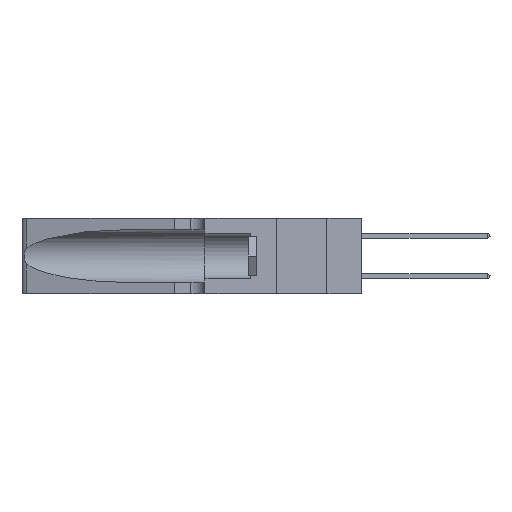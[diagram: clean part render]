
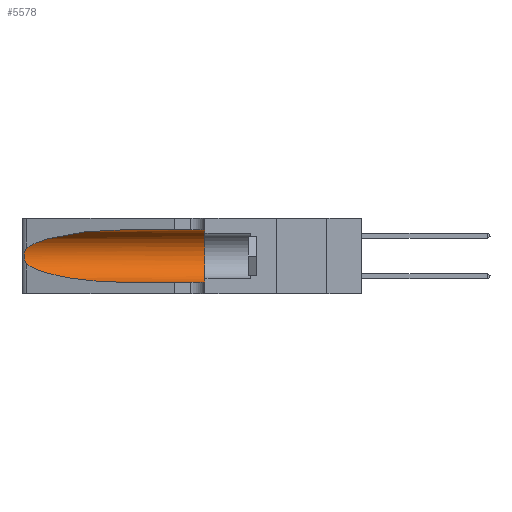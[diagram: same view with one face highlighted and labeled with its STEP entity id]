
A CAD part, left-side view. The second image highlights one B-rep face of the part: STEP entity #5578.
In plain terms, the highlighted cylindrical face has radius 3.308 mm (diameter 6.617 mm), a partial arc.
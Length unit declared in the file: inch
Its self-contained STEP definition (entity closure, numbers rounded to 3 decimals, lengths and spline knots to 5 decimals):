
#259 = CARTESIAN_POINT ( 'NONE',  ( 0.26075, 1.23896, 0.19203 ) ) ;
#334 = VERTEX_POINT ( 'NONE', #24990 ) ;
#492 = CARTESIAN_POINT ( 'NONE',  ( 0.25487, 1.22718, 0.22369 ) ) ;
#1660 = ORIENTED_EDGE ( 'NONE', *, *, #24287, .T. ) ;
#2273 = CARTESIAN_POINT ( 'NONE',  ( 0.25555, 1.22994, 0.2215 ) ) ;
#2366 = CARTESIAN_POINT ( 'NONE',  ( 0.26017, 1.23833, 0.17102 ) ) ;
#2675 = CARTESIAN_POINT ( 'NONE',  ( 0.25487, 1.22718, 0.14631 ) ) ;
#3434 = VERTEX_POINT ( 'NONE', #2675 ) ;
#4401 = CARTESIAN_POINT ( 'NONE',  ( 0.25487, 1.22718, 0.22369 ) ) ;
#4491 = CARTESIAN_POINT ( 'NONE',  ( 0.25789, 1.23486, 0.15765 ) ) ;
#5123 = VECTOR ( 'NONE', #13664, 39.37008 ) ;
#5188 = DIRECTION ( 'NONE',  ( 0., -1., 0. ) ) ;
#5388 = CARTESIAN_POINT ( 'NONE',  ( 0.1305, 0.35, 0.05475 ) ) ;
#5578 = ADVANCED_FACE ( 'NONE', ( #5948 ), #21377, .F. ) ;
#5700 = ORIENTED_EDGE ( 'NONE', *, *, #9911, .T. ) ;
#5877 = VERTEX_POINT ( 'NONE', #492 ) ;
#5948 = FACE_OUTER_BOUND ( 'NONE', #6174, .T. ) ;
#6094 = ORIENTED_EDGE ( 'NONE', *, *, #17250, .F. ) ;
#6174 = EDGE_LOOP ( 'NONE', ( #10050, #5700, #1660, #6960, #9181, #6094 ) ) ;
#6237 =( BOUNDED_CURVE ( )  B_SPLINE_CURVE ( 3, ( #12435, #24240, #20413, #8373 ),
 .UNSPECIFIED., .F., .F. ) 
 B_SPLINE_CURVE_WITH_KNOTS ( ( 4, 4 ),
 ( 3.44316, 4.71239 ),
 .UNSPECIFIED. ) 
 CURVE ( )  GEOMETRIC_REPRESENTATION_ITEM ( )  RATIONAL_B_SPLINE_CURVE ( ( 1., 0.87, 0.87, 1. ) ) 
 REPRESENTATION_ITEM ( '' )  );
#6446 = LINE ( 'NONE', #23230, #17261 ) ;
#6605 = CARTESIAN_POINT ( 'NONE',  ( 0.25555, 1.22993, 0.14849 ) ) ;
#6960 = ORIENTED_EDGE ( 'NONE', *, *, #17179, .T. ) ;
#6998 = AXIS2_PLACEMENT_3D ( 'NONE', #14199, #18118, #25963 ) ;
#8162 = CARTESIAN_POINT ( 'NONE',  ( 0.18966, 0.96281, 0.31525 ) ) ;
#8370 = VERTEX_POINT ( 'NONE', #22132 ) ;
#8373 = CARTESIAN_POINT ( 'NONE',  ( 0.1305, 0.72297, 0.05475 ) ) ;
#9181 = ORIENTED_EDGE ( 'NONE', *, *, #9802, .F. ) ;
#9802 = EDGE_CURVE ( 'NONE', #334, #20922, #17968, .T. ) ;
#9911 = EDGE_CURVE ( 'NONE', #5877, #3434, #17657, .T. ) ;
#10050 = ORIENTED_EDGE ( 'NONE', *, *, #18029, .T. ) ;
#10668 = CARTESIAN_POINT ( 'NONE',  ( 0.25787, 1.23484, 0.2124 ) ) ;
#12302 = CARTESIAN_POINT ( 'NONE',  ( 0.25487, 1.22718, 0.22369 ) ) ;
#12375 = CARTESIAN_POINT ( 'NONE',  ( 0.1305, 0.35, 0.185 ) ) ;
#12435 = CARTESIAN_POINT ( 'NONE',  ( 0.25487, 1.22718, 0.14631 ) ) ;
#12731 = CARTESIAN_POINT ( 'NONE',  ( 0.26018, 1.23835, 0.19895 ) ) ;
#13664 = DIRECTION ( 'NONE',  ( 0., -1., 0. ) ) ;
#14199 = CARTESIAN_POINT ( 'NONE',  ( 0.1305, 1.61858, 0.185 ) ) ;
#14398 = DIRECTION ( 'NONE',  ( 0., 0., 1. ) ) ;
#14737 = CARTESIAN_POINT ( 'NONE',  ( 0.26075, 1.23896, 0.178 ) ) ;
#14792 = CARTESIAN_POINT ( 'NONE',  ( 0.1305, 0.72297, 0.05475 ) ) ;
#16740 = CARTESIAN_POINT ( 'NONE',  ( 0.25856, 1.23593, 0.16098 ) ) ;
#16981 = VERTEX_POINT ( 'NONE', #14792 ) ;
#17179 = EDGE_CURVE ( 'NONE', #16981, #20922, #6446, .T. ) ;
#17250 = EDGE_CURVE ( 'NONE', #8370, #334, #25206, .T. ) ;
#17261 = VECTOR ( 'NONE', #5188, 39.37008 ) ;
#17657 = B_SPLINE_CURVE_WITH_KNOTS ( 'NONE', 3,
 ( #4401, #2273, #22573, #10668, #24519, #12731, #259, #14737, #2366, #16740, #4491, #18718, #6605, #20693 ),
 .UNSPECIFIED., .F., .F.,
 ( 4, 2, 2, 2, 2, 2, 4 ),
 ( 0., 0.00027, 0.00053, 0.00107, 0.0016, 0.00187, 0.00214 ),
 .UNSPECIFIED. ) ;
#17968 = CIRCLE ( 'NONE', #25612, 0.13025 ) ;
#18029 = EDGE_CURVE ( 'NONE', #8370, #5877, #24833, .T. ) ;
#18118 = DIRECTION ( 'NONE',  ( 0., -1., 0. ) ) ;
#18718 = CARTESIAN_POINT ( 'NONE',  ( 0.25639, 1.23186, 0.15144 ) ) ;
#20413 = CARTESIAN_POINT ( 'NONE',  ( 0.18966, 0.96281, 0.05475 ) ) ;
#20693 = CARTESIAN_POINT ( 'NONE',  ( 0.25487, 1.22718, 0.14631 ) ) ;
#20922 = VERTEX_POINT ( 'NONE', #5388 ) ;
#21377 = CYLINDRICAL_SURFACE ( 'NONE', #6998, 0.13025 ) ;
#22132 = CARTESIAN_POINT ( 'NONE',  ( 0.1305, 0.72297, 0.31525 ) ) ;
#22163 = CARTESIAN_POINT ( 'NONE',  ( 0.1305, 0.72297, 0.31525 ) ) ;
#22573 = CARTESIAN_POINT ( 'NONE',  ( 0.25639, 1.23184, 0.21858 ) ) ;
#23230 = CARTESIAN_POINT ( 'NONE',  ( 0.1305, 1.61858, 0.05475 ) ) ;
#24120 = CARTESIAN_POINT ( 'NONE',  ( 0.2373, 1.15595, 0.28018 ) ) ;
#24240 = CARTESIAN_POINT ( 'NONE',  ( 0.2373, 1.15595, 0.08982 ) ) ;
#24287 = EDGE_CURVE ( 'NONE', #3434, #16981, #6237, .T. ) ;
#24519 = CARTESIAN_POINT ( 'NONE',  ( 0.25854, 1.2359, 0.20912 ) ) ;
#24833 =( BOUNDED_CURVE ( )  B_SPLINE_CURVE ( 3, ( #22163, #8162, #24120, #12302 ),
 .UNSPECIFIED., .F., .F. ) 
 B_SPLINE_CURVE_WITH_KNOTS ( ( 4, 4 ),
 ( 1.5708, 2.84003 ),
 .UNSPECIFIED. ) 
 CURVE ( )  GEOMETRIC_REPRESENTATION_ITEM ( )  RATIONAL_B_SPLINE_CURVE ( ( 1., 0.87, 0.87, 1. ) ) 
 REPRESENTATION_ITEM ( '' )  );
#24990 = CARTESIAN_POINT ( 'NONE',  ( 0.1305, 0.35, 0.31525 ) ) ;
#25206 = LINE ( 'NONE', #25421, #5123 ) ;
#25421 = CARTESIAN_POINT ( 'NONE',  ( 0.1305, 1.61858, 0.31525 ) ) ;
#25612 = AXIS2_PLACEMENT_3D ( 'NONE', #12375, #26155, #14398 ) ;
#25963 = DIRECTION ( 'NONE',  ( 0., 0., -1. ) ) ;
#26155 = DIRECTION ( 'NONE',  ( 0., 1., 0. ) ) ;
